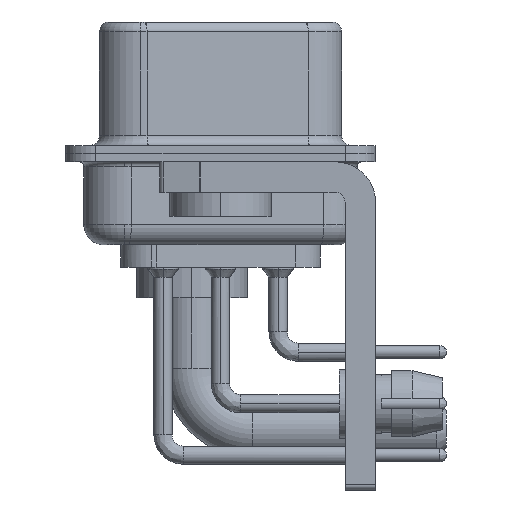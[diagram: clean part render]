
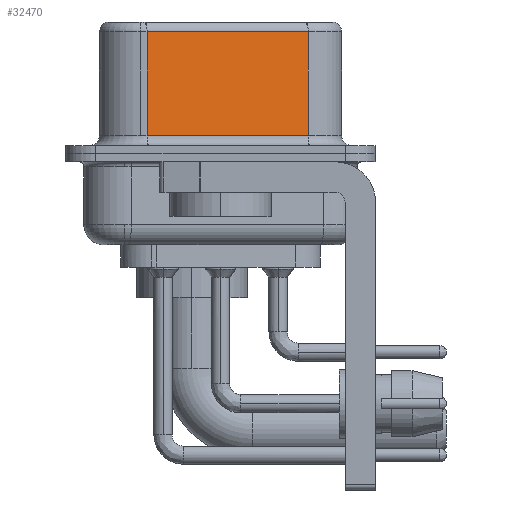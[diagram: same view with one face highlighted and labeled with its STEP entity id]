
A CAD part, left-side view. The second image highlights one B-rep face of the part: STEP entity #32470.
In plain terms, the highlighted planar face has unit normal (-0.985, -0.174, 0).
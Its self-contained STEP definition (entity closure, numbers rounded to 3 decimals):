
#847 = VECTOR ( 'NONE', #33615, 1000. ) ;
#1144 = DIRECTION ( 'NONE',  ( 0.985, 0.174, 0. ) ) ;
#2237 = VERTEX_POINT ( 'NONE', #30594 ) ;
#2625 = DIRECTION ( 'NONE',  ( 0., 0., -1. ) ) ;
#3301 = DIRECTION ( 'NONE',  ( -0.174, 0.985, 0. ) ) ;
#3478 = ORIENTED_EDGE ( 'NONE', *, *, #10918, .T. ) ;
#3589 = EDGE_CURVE ( 'NONE', #10307, #36098, #30602, .T. ) ;
#4567 = DIRECTION ( 'NONE',  ( -0.174, 0.985, 0. ) ) ;
#6265 = ORIENTED_EDGE ( 'NONE', *, *, #38658, .F. ) ;
#8071 = CARTESIAN_POINT ( 'NONE',  ( 3.73, 3.628, 0.9 ) ) ;
#10209 = ORIENTED_EDGE ( 'NONE', *, *, #37770, .T. ) ;
#10307 = VERTEX_POINT ( 'NONE', #16920 ) ;
#10918 = EDGE_CURVE ( 'NONE', #30351, #2237, #18063, .T. ) ;
#12343 = CARTESIAN_POINT ( 'NONE',  ( 5.132, -4.322, 6.52 ) ) ;
#13010 = VECTOR ( 'NONE', #2625, 1000. ) ;
#13457 = VECTOR ( 'NONE', #3301, 1000. ) ;
#14319 = LINE ( 'NONE', #33161, #13010 ) ;
#16483 = FACE_OUTER_BOUND ( 'NONE', #17889, .T. ) ;
#16920 = CARTESIAN_POINT ( 'NONE',  ( 5.132, -4.322, 6.02 ) ) ;
#17889 = EDGE_LOOP ( 'NONE', ( #6265, #18787, #10209, #3478 ) ) ;
#18063 = LINE ( 'NONE', #39724, #27794 ) ;
#18787 = ORIENTED_EDGE ( 'NONE', *, *, #3589, .T. ) ;
#24540 = CARTESIAN_POINT ( 'NONE',  ( 5.132, -4.322, 6.02 ) ) ;
#27346 = LINE ( 'NONE', #12343, #847 ) ;
#27794 = VECTOR ( 'NONE', #30413, 1000. ) ;
#28839 = PLANE ( 'NONE',  #38630 ) ;
#29360 = CARTESIAN_POINT ( 'NONE',  ( 3.73, 3.628, 6.02 ) ) ;
#30351 = VERTEX_POINT ( 'NONE', #8071 ) ;
#30413 = DIRECTION ( 'NONE',  ( 0.174, -0.985, 0. ) ) ;
#30594 = CARTESIAN_POINT ( 'NONE',  ( 5.132, -4.322, 0.9 ) ) ;
#30602 = LINE ( 'NONE', #24540, #13457 ) ;
#32470 = ADVANCED_FACE ( 'NONE', ( #16483 ), #28839, .F. ) ;
#33161 = CARTESIAN_POINT ( 'NONE',  ( 3.73, 3.628, 6.52 ) ) ;
#33615 = DIRECTION ( 'NONE',  ( 0., 0., -1. ) ) ;
#36098 = VERTEX_POINT ( 'NONE', #29360 ) ;
#37770 = EDGE_CURVE ( 'NONE', #36098, #30351, #14319, .T. ) ;
#38344 = CARTESIAN_POINT ( 'NONE',  ( 5.132, -4.322, 6.52 ) ) ;
#38630 = AXIS2_PLACEMENT_3D ( 'NONE', #38344, #1144, #4567 ) ;
#38658 = EDGE_CURVE ( 'NONE', #10307, #2237, #27346, .T. ) ;
#39724 = CARTESIAN_POINT ( 'NONE',  ( 5.132, -4.322, 0.9 ) ) ;
